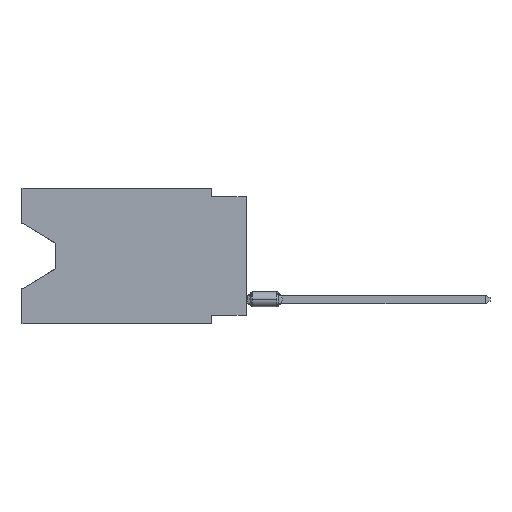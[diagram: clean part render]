
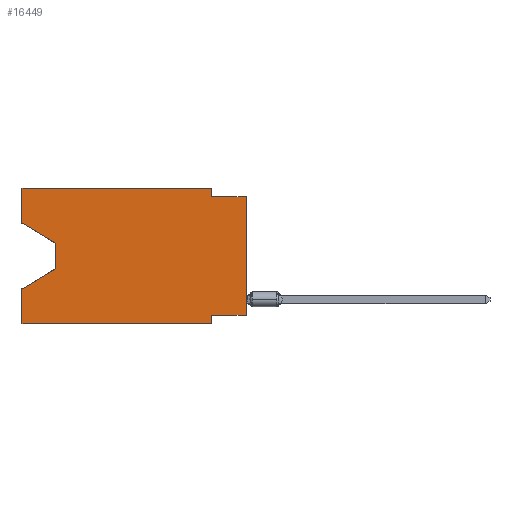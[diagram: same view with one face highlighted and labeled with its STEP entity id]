
A CAD part, left-side view. The second image highlights one B-rep face of the part: STEP entity #16449.
In plain terms, the highlighted planar face has unit normal (-1, 0, 0).
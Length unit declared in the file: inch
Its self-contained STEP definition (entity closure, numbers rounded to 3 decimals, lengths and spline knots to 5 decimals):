
#230 = EDGE_CURVE ( 'NONE', #2845, #1108, #20131, .T. ) ;
#326 = CARTESIAN_POINT ( 'NONE',  ( 0., 0.1, -0.39 ) ) ;
#619 = VERTEX_POINT ( 'NONE', #326 ) ;
#1050 = VECTOR ( 'NONE', #7994, 39.37008 ) ;
#1108 = VERTEX_POINT ( 'NONE', #20777 ) ;
#1692 = LINE ( 'NONE', #13066, #10553 ) ;
#1805 = DIRECTION ( 'NONE',  ( 0., 0., 1. ) ) ;
#2043 = CARTESIAN_POINT ( 'NONE',  ( 0., 0.1, 0. ) ) ;
#2568 = CARTESIAN_POINT ( 'NONE',  ( 0., 0.645, -0.39 ) ) ;
#2845 = VERTEX_POINT ( 'NONE', #7730 ) ;
#2938 = VERTEX_POINT ( 'NONE', #15660 ) ;
#3198 = CARTESIAN_POINT ( 'NONE',  ( 0., 0.645, -0.28975 ) ) ;
#3261 = DIRECTION ( 'NONE',  ( 0., 1., 0. ) ) ;
#3339 = LINE ( 'NONE', #14800, #16091 ) ;
#3423 = EDGE_CURVE ( 'NONE', #10935, #9001, #1692, .T. ) ;
#3683 = CARTESIAN_POINT ( 'NONE',  ( 0., 0.55, -0.232 ) ) ;
#4001 = LINE ( 'NONE', #7827, #16539 ) ;
#4060 = LINE ( 'NONE', #2568, #14810 ) ;
#4084 = CARTESIAN_POINT ( 'NONE',  ( 0., 0., -0.025 ) ) ;
#4112 = EDGE_CURVE ( 'NONE', #10935, #13448, #6335, .T. ) ;
#4361 = LINE ( 'NONE', #17527, #1050 ) ;
#4480 = CARTESIAN_POINT ( 'NONE',  ( 0., 0.645, 0. ) ) ;
#4957 = CARTESIAN_POINT ( 'NONE',  ( 0., 0., -0.365 ) ) ;
#5095 = LINE ( 'NONE', #15825, #11369 ) ;
#5258 = DIRECTION ( 'NONE',  ( 0., 0., -1. ) ) ;
#5362 = VERTEX_POINT ( 'NONE', #12812 ) ;
#5544 = VECTOR ( 'NONE', #17780, 39.37008 ) ;
#5598 = ORIENTED_EDGE ( 'NONE', *, *, #12036, .F. ) ;
#5630 = DIRECTION ( 'NONE',  ( 0., -1., 0. ) ) ;
#5715 = ORIENTED_EDGE ( 'NONE', *, *, #19867, .F. ) ;
#6080 = FACE_OUTER_BOUND ( 'NONE', #18619, .T. ) ;
#6250 = CARTESIAN_POINT ( 'NONE',  ( 0., 0., -0.365 ) ) ;
#6335 = LINE ( 'NONE', #4957, #20145 ) ;
#6766 = LINE ( 'NONE', #3683, #10726 ) ;
#6927 = DIRECTION ( 'NONE',  ( 0., 0., -1. ) ) ;
#7033 = EDGE_CURVE ( 'NONE', #13448, #619, #4361, .T. ) ;
#7654 = CARTESIAN_POINT ( 'NONE',  ( 0., 0.645, -0.10025 ) ) ;
#7730 = CARTESIAN_POINT ( 'NONE',  ( 0., 0.55, -0.158 ) ) ;
#7827 = CARTESIAN_POINT ( 'NONE',  ( 0., 0.645, 0. ) ) ;
#7994 = DIRECTION ( 'NONE',  ( 0., 0., -1. ) ) ;
#8076 = DIRECTION ( 'NONE',  ( 0., -1., 0. ) ) ;
#8106 = ORIENTED_EDGE ( 'NONE', *, *, #230, .T. ) ;
#8358 = CARTESIAN_POINT ( 'NONE',  ( 0., 0.645, 0. ) ) ;
#8651 = LINE ( 'NONE', #2043, #15775 ) ;
#9001 = VERTEX_POINT ( 'NONE', #4084 ) ;
#9049 = DIRECTION ( 'NONE',  ( 0., -1., 0. ) ) ;
#9091 = DIRECTION ( 'NONE',  ( 0., 0., 1. ) ) ;
#9380 = DIRECTION ( 'NONE',  ( 1., 0., 0. ) ) ;
#9808 = DIRECTION ( 'NONE',  ( 0., -0.855, -0.519 ) ) ;
#10011 = VERTEX_POINT ( 'NONE', #7654 ) ;
#10310 = LINE ( 'NONE', #13894, #17514 ) ;
#10345 = CARTESIAN_POINT ( 'NONE',  ( 0., 0.55, -0.158 ) ) ;
#10553 = VECTOR ( 'NONE', #1805, 39.37008 ) ;
#10726 = VECTOR ( 'NONE', #19627, 39.37008 ) ;
#10935 = VERTEX_POINT ( 'NONE', #6250 ) ;
#11165 = CARTESIAN_POINT ( 'NONE',  ( 0., 0.1, -0.365 ) ) ;
#11369 = VECTOR ( 'NONE', #8076, 39.37008 ) ;
#11611 = EDGE_CURVE ( 'NONE', #1108, #18209, #6766, .T. ) ;
#11911 = ORIENTED_EDGE ( 'NONE', *, *, #7033, .F. ) ;
#12036 = EDGE_CURVE ( 'NONE', #5362, #14707, #8651, .T. ) ;
#12217 = EDGE_CURVE ( 'NONE', #13538, #5362, #5095, .T. ) ;
#12551 = PLANE ( 'NONE',  #18106 ) ;
#12739 = CARTESIAN_POINT ( 'NONE',  ( 0., 0.645, 0. ) ) ;
#12812 = CARTESIAN_POINT ( 'NONE',  ( 0., 0.1, 0. ) ) ;
#12849 = ORIENTED_EDGE ( 'NONE', *, *, #13665, .F. ) ;
#13066 = CARTESIAN_POINT ( 'NONE',  ( 0., 0., 0. ) ) ;
#13354 = EDGE_CURVE ( 'NONE', #2938, #619, #4060, .T. ) ;
#13366 = VECTOR ( 'NONE', #5258, 39.37008 ) ;
#13405 = ORIENTED_EDGE ( 'NONE', *, *, #4112, .F. ) ;
#13448 = VERTEX_POINT ( 'NONE', #11165 ) ;
#13538 = VERTEX_POINT ( 'NONE', #12739 ) ;
#13665 = EDGE_CURVE ( 'NONE', #14707, #9001, #10310, .T. ) ;
#13894 = CARTESIAN_POINT ( 'NONE',  ( 0., 0., -0.025 ) ) ;
#14187 = ORIENTED_EDGE ( 'NONE', *, *, #17802, .T. ) ;
#14707 = VERTEX_POINT ( 'NONE', #19144 ) ;
#14718 = LINE ( 'NONE', #8358, #5544 ) ;
#14800 = CARTESIAN_POINT ( 'NONE',  ( 0., 0.645, -0.10025 ) ) ;
#14810 = VECTOR ( 'NONE', #9049, 39.37008 ) ;
#14948 = ORIENTED_EDGE ( 'NONE', *, *, #16093, .F. ) ;
#15034 = ORIENTED_EDGE ( 'NONE', *, *, #11611, .T. ) ;
#15660 = CARTESIAN_POINT ( 'NONE',  ( 0., 0.645, -0.39 ) ) ;
#15775 = VECTOR ( 'NONE', #19808, 39.37008 ) ;
#15825 = CARTESIAN_POINT ( 'NONE',  ( 0., 0.645, 0. ) ) ;
#16091 = VECTOR ( 'NONE', #9808, 39.37008 ) ;
#16093 = EDGE_CURVE ( 'NONE', #10011, #13538, #14718, .T. ) ;
#16449 = ADVANCED_FACE ( 'NONE', ( #6080 ), #12551, .F. ) ;
#16539 = VECTOR ( 'NONE', #9091, 39.37008 ) ;
#17297 = ORIENTED_EDGE ( 'NONE', *, *, #12217, .F. ) ;
#17514 = VECTOR ( 'NONE', #5630, 39.37008 ) ;
#17527 = CARTESIAN_POINT ( 'NONE',  ( 0., 0.1, -0.39 ) ) ;
#17780 = DIRECTION ( 'NONE',  ( 0., 0., 1. ) ) ;
#17802 = EDGE_CURVE ( 'NONE', #10011, #2845, #3339, .T. ) ;
#18106 = AXIS2_PLACEMENT_3D ( 'NONE', #4480, #9380, #6927 ) ;
#18209 = VERTEX_POINT ( 'NONE', #3198 ) ;
#18230 = ORIENTED_EDGE ( 'NONE', *, *, #13354, .T. ) ;
#18619 = EDGE_LOOP ( 'NONE', ( #14187, #8106, #15034, #5715, #18230, #11911, #13405, #19091, #12849, #5598, #17297, #14948 ) ) ;
#19091 = ORIENTED_EDGE ( 'NONE', *, *, #3423, .T. ) ;
#19144 = CARTESIAN_POINT ( 'NONE',  ( 0., 0.1, -0.025 ) ) ;
#19627 = DIRECTION ( 'NONE',  ( 0., 0.855, -0.519 ) ) ;
#19808 = DIRECTION ( 'NONE',  ( 0., 0., -1. ) ) ;
#19867 = EDGE_CURVE ( 'NONE', #2938, #18209, #4001, .T. ) ;
#20131 = LINE ( 'NONE', #10345, #13366 ) ;
#20145 = VECTOR ( 'NONE', #3261, 39.37008 ) ;
#20777 = CARTESIAN_POINT ( 'NONE',  ( 0., 0.55, -0.232 ) ) ;
